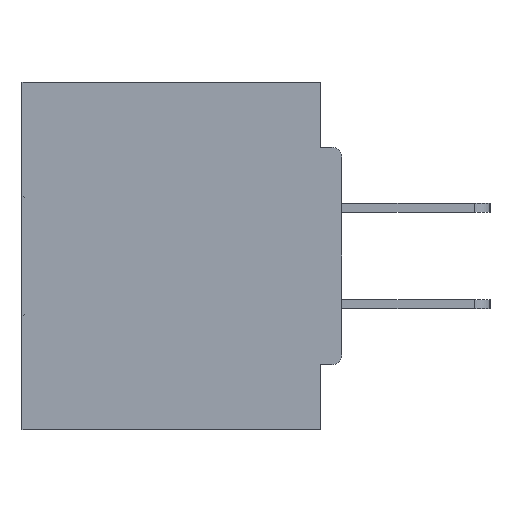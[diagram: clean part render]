
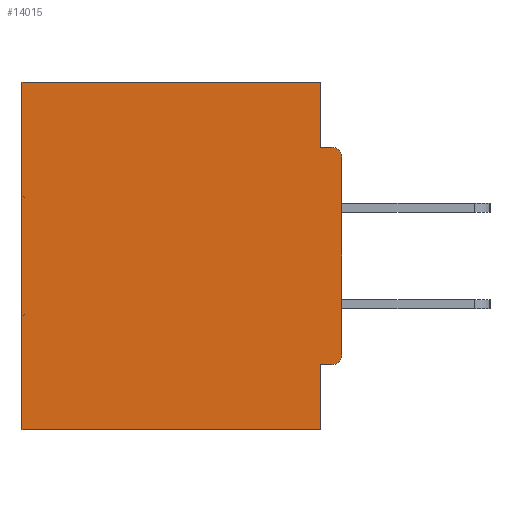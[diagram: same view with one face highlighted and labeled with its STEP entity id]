
A CAD part, left-side view. The second image highlights one B-rep face of the part: STEP entity #14015.
In plain terms, the highlighted planar face has unit normal (-1, 0, 0).
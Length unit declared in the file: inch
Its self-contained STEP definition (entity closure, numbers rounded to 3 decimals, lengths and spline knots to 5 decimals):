
#2031 = CARTESIAN_POINT ( 'NONE',  ( 0.298, 0., -0.0935 ) ) ;
#2167 = CARTESIAN_POINT ( 'NONE',  ( 0.298, 0., 0. ) ) ;
#2417 = CARTESIAN_POINT ( 'NONE',  ( 0.298, 0., -0.4065 ) ) ;
#2783 = VERTEX_POINT ( 'NONE', #21762 ) ;
#3944 = CARTESIAN_POINT ( 'NONE',  ( 0.298, 0., 0. ) ) ;
#4276 = ORIENTED_EDGE ( 'NONE', *, *, #15728, .F. ) ;
#4633 = VECTOR ( 'NONE', #18842, 39.37008 ) ;
#4685 = VECTOR ( 'NONE', #42205, 39.37008 ) ;
#4817 = CARTESIAN_POINT ( 'NONE',  ( 0.298, 0., -0.5 ) ) ;
#5018 = DIRECTION ( 'NONE',  ( 0., 0., -1. ) ) ;
#5027 = VECTOR ( 'NONE', #12438, 39.37008 ) ;
#5413 = VERTEX_POINT ( 'NONE', #28122 ) ;
#5446 = DIRECTION ( 'NONE',  ( 0., 0., -1. ) ) ;
#5628 = CARTESIAN_POINT ( 'NONE',  ( 0.298, 0.015, -0.4065 ) ) ;
#5933 = EDGE_CURVE ( 'NONE', #27429, #2783, #9910, .T. ) ;
#6278 = EDGE_CURVE ( 'NONE', #27310, #40341, #37122, .T. ) ;
#6698 = LINE ( 'NONE', #2031, #17929 ) ;
#7046 = AXIS2_PLACEMENT_3D ( 'NONE', #22058, #35112, #5018 ) ;
#7292 = LINE ( 'NONE', #39669, #26485 ) ;
#7730 = EDGE_CURVE ( 'NONE', #11543, #42922, #36954, .T. ) ;
#8081 = ORIENTED_EDGE ( 'NONE', *, *, #42864, .F. ) ;
#8367 = DIRECTION ( 'NONE',  ( 0., 0., -1. ) ) ;
#8820 = DIRECTION ( 'NONE',  ( 0., 1., 0. ) ) ;
#9651 = CIRCLE ( 'NONE', #7046, 0.015 ) ;
#9910 = CIRCLE ( 'NONE', #34844, 0.015 ) ;
#10481 = LINE ( 'NONE', #32060, #4633 ) ;
#11333 = VERTEX_POINT ( 'NONE', #25414 ) ;
#11543 = VERTEX_POINT ( 'NONE', #27984 ) ;
#12221 = DIRECTION ( 'NONE',  ( -1., 0., 0. ) ) ;
#12438 = DIRECTION ( 'NONE',  ( 0., 0., -1. ) ) ;
#12683 = DIRECTION ( 'NONE',  ( 0., 1., 0. ) ) ;
#14015 = ADVANCED_FACE ( 'NONE', ( #18653 ), #16022, .F. ) ;
#15008 = VERTEX_POINT ( 'NONE', #37890 ) ;
#15096 = AXIS2_PLACEMENT_3D ( 'NONE', #2167, #29584, #23088 ) ;
#15728 = EDGE_CURVE ( 'NONE', #35360, #15008, #6698, .T. ) ;
#16022 = PLANE ( 'NONE',  #15096 ) ;
#17748 = EDGE_CURVE ( 'NONE', #27429, #27310, #37995, .T. ) ;
#17929 = VECTOR ( 'NONE', #39685, 39.37008 ) ;
#18476 = CARTESIAN_POINT ( 'NONE',  ( 0.298, 0.031, -0.0935 ) ) ;
#18645 = CARTESIAN_POINT ( 'NONE',  ( 0.298, 0.031, -0.4065 ) ) ;
#18653 = FACE_OUTER_BOUND ( 'NONE', #33319, .T. ) ;
#18842 = DIRECTION ( 'NONE',  ( 0., 1., 0. ) ) ;
#21762 = CARTESIAN_POINT ( 'NONE',  ( 0.298, 0., -0.3915 ) ) ;
#21983 = ORIENTED_EDGE ( 'NONE', *, *, #5933, .T. ) ;
#22058 = CARTESIAN_POINT ( 'NONE',  ( 0.298, 0.015, -0.1085 ) ) ;
#23088 = DIRECTION ( 'NONE',  ( 0., 0., -1. ) ) ;
#23721 = ORIENTED_EDGE ( 'NONE', *, *, #7730, .T. ) ;
#24468 = LINE ( 'NONE', #4817, #32376 ) ;
#24469 = ORIENTED_EDGE ( 'NONE', *, *, #17748, .F. ) ;
#25308 = CARTESIAN_POINT ( 'NONE',  ( 0.298, 0.031, -0.5 ) ) ;
#25414 = CARTESIAN_POINT ( 'NONE',  ( 0.298, 0.031, 0. ) ) ;
#25959 = DIRECTION ( 'NONE',  ( 0., 0., -1. ) ) ;
#26485 = VECTOR ( 'NONE', #5446, 39.37008 ) ;
#26541 = ORIENTED_EDGE ( 'NONE', *, *, #42212, .F. ) ;
#27310 = VERTEX_POINT ( 'NONE', #18645 ) ;
#27429 = VERTEX_POINT ( 'NONE', #5628 ) ;
#27984 = CARTESIAN_POINT ( 'NONE',  ( 0.298, 0.46, 0. ) ) ;
#28122 = CARTESIAN_POINT ( 'NONE',  ( 0.298, 0., -0.1085 ) ) ;
#29207 = CARTESIAN_POINT ( 'NONE',  ( 0.298, 0.015, -0.3915 ) ) ;
#29284 = CARTESIAN_POINT ( 'NONE',  ( 0.298, 0.46, 0. ) ) ;
#29584 = DIRECTION ( 'NONE',  ( 1., 0., 0. ) ) ;
#30157 = ORIENTED_EDGE ( 'NONE', *, *, #37720, .T. ) ;
#32060 = CARTESIAN_POINT ( 'NONE',  ( 0.298, 0., 0. ) ) ;
#32072 = ORIENTED_EDGE ( 'NONE', *, *, #32220, .F. ) ;
#32220 = EDGE_CURVE ( 'NONE', #5413, #2783, #36118, .T. ) ;
#32376 = VECTOR ( 'NONE', #8820, 39.37008 ) ;
#32757 = ORIENTED_EDGE ( 'NONE', *, *, #6278, .F. ) ;
#33184 = VECTOR ( 'NONE', #12683, 39.37008 ) ;
#33319 = EDGE_LOOP ( 'NONE', ( #35177, #4276, #8081, #30157, #23721, #26541, #32757, #24469, #21983, #32072 ) ) ;
#34844 = AXIS2_PLACEMENT_3D ( 'NONE', #29207, #12221, #8367 ) ;
#35112 = DIRECTION ( 'NONE',  ( -1., 0., 0. ) ) ;
#35177 = ORIENTED_EDGE ( 'NONE', *, *, #40354, .T. ) ;
#35360 = VERTEX_POINT ( 'NONE', #18476 ) ;
#36082 = VECTOR ( 'NONE', #25959, 39.37008 ) ;
#36118 = LINE ( 'NONE', #3944, #4685 ) ;
#36406 = CARTESIAN_POINT ( 'NONE',  ( 0.298, 0.46, -0.5 ) ) ;
#36954 = LINE ( 'NONE', #29284, #5027 ) ;
#37122 = LINE ( 'NONE', #38449, #36082 ) ;
#37720 = EDGE_CURVE ( 'NONE', #11333, #11543, #10481, .T. ) ;
#37890 = CARTESIAN_POINT ( 'NONE',  ( 0.298, 0.015, -0.0935 ) ) ;
#37995 = LINE ( 'NONE', #2417, #33184 ) ;
#38449 = CARTESIAN_POINT ( 'NONE',  ( 0.298, 0.031, -0.5 ) ) ;
#39669 = CARTESIAN_POINT ( 'NONE',  ( 0.298, 0.031, -0.5 ) ) ;
#39685 = DIRECTION ( 'NONE',  ( 0., -1., 0. ) ) ;
#40341 = VERTEX_POINT ( 'NONE', #25308 ) ;
#40354 = EDGE_CURVE ( 'NONE', #5413, #15008, #9651, .T. ) ;
#42205 = DIRECTION ( 'NONE',  ( 0., 0., -1. ) ) ;
#42212 = EDGE_CURVE ( 'NONE', #40341, #42922, #24468, .T. ) ;
#42864 = EDGE_CURVE ( 'NONE', #11333, #35360, #7292, .T. ) ;
#42922 = VERTEX_POINT ( 'NONE', #36406 ) ;
